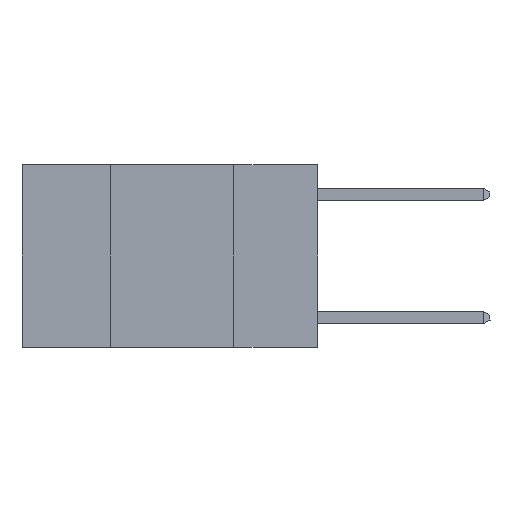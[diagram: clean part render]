
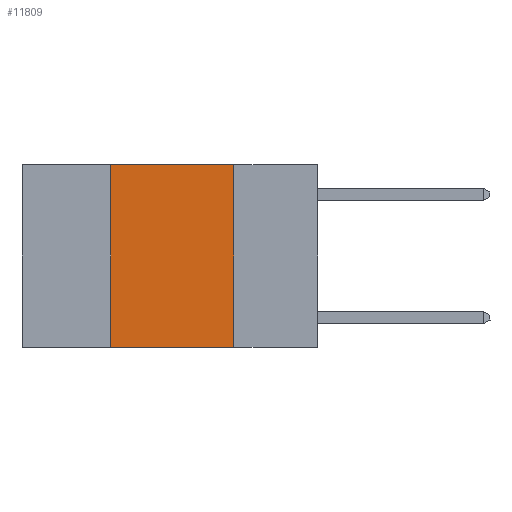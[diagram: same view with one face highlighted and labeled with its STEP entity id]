
A CAD part, left-side view. The second image highlights one B-rep face of the part: STEP entity #11809.
In plain terms, the highlighted planar face has unit normal (-1, 0, 0).
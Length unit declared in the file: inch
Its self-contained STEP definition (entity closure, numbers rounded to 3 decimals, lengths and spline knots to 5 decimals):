
#239 = CARTESIAN_POINT ( 'NONE',  ( 0., 0.6, 0. ) ) ;
#1172 = EDGE_CURVE ( 'NONE', #4016, #11119, #20308, .T. ) ;
#1400 = VECTOR ( 'NONE', #7368, 39.37008 ) ;
#1978 = EDGE_LOOP ( 'NONE', ( #10101, #2182, #15160, #20377 ) ) ;
#2021 = CARTESIAN_POINT ( 'NONE',  ( 0., 0.17, 0. ) ) ;
#2182 = ORIENTED_EDGE ( 'NONE', *, *, #1172, .F. ) ;
#2246 = CARTESIAN_POINT ( 'NONE',  ( 0., 0.42, 0. ) ) ;
#2479 = CARTESIAN_POINT ( 'NONE',  ( 0., 0.17, 0. ) ) ;
#2783 = LINE ( 'NONE', #2479, #1400 ) ;
#4016 = VERTEX_POINT ( 'NONE', #2246 ) ;
#6223 = VECTOR ( 'NONE', #20304, 39.37008 ) ;
#6558 = CARTESIAN_POINT ( 'NONE',  ( 0., 0.17, -0.37 ) ) ;
#6896 = EDGE_CURVE ( 'NONE', #16658, #4016, #13986, .T. ) ;
#7368 = DIRECTION ( 'NONE',  ( 0., 0., -1. ) ) ;
#7430 = AXIS2_PLACEMENT_3D ( 'NONE', #239, #19223, #14659 ) ;
#8344 = FACE_OUTER_BOUND ( 'NONE', #1978, .T. ) ;
#8404 = LINE ( 'NONE', #17831, #14556 ) ;
#9434 = CARTESIAN_POINT ( 'NONE',  ( 0., 0.6, 0. ) ) ;
#9654 = VECTOR ( 'NONE', #15734, 39.37008 ) ;
#10101 = ORIENTED_EDGE ( 'NONE', *, *, #17708, .F. ) ;
#10576 = CARTESIAN_POINT ( 'NONE',  ( 0., 0.42, 0. ) ) ;
#11119 = VERTEX_POINT ( 'NONE', #2021 ) ;
#11591 = CARTESIAN_POINT ( 'NONE',  ( 0., 0.42, -0.37 ) ) ;
#11809 = ADVANCED_FACE ( 'NONE', ( #8344 ), #15899, .F. ) ;
#13679 = VERTEX_POINT ( 'NONE', #6558 ) ;
#13986 = LINE ( 'NONE', #10576, #6223 ) ;
#14556 = VECTOR ( 'NONE', #17522, 39.37008 ) ;
#14659 = DIRECTION ( 'NONE',  ( 0., 0., -1. ) ) ;
#15160 = ORIENTED_EDGE ( 'NONE', *, *, #6896, .F. ) ;
#15734 = DIRECTION ( 'NONE',  ( 0., -1., 0. ) ) ;
#15899 = PLANE ( 'NONE',  #7430 ) ;
#16166 = EDGE_CURVE ( 'NONE', #16658, #13679, #8404, .T. ) ;
#16658 = VERTEX_POINT ( 'NONE', #11591 ) ;
#17522 = DIRECTION ( 'NONE',  ( 0., -1., 0. ) ) ;
#17708 = EDGE_CURVE ( 'NONE', #11119, #13679, #2783, .T. ) ;
#17831 = CARTESIAN_POINT ( 'NONE',  ( 0., 0.6, -0.37 ) ) ;
#19223 = DIRECTION ( 'NONE',  ( 1., 0., 0. ) ) ;
#20304 = DIRECTION ( 'NONE',  ( 0., 0., 1. ) ) ;
#20308 = LINE ( 'NONE', #9434, #9654 ) ;
#20377 = ORIENTED_EDGE ( 'NONE', *, *, #16166, .T. ) ;
